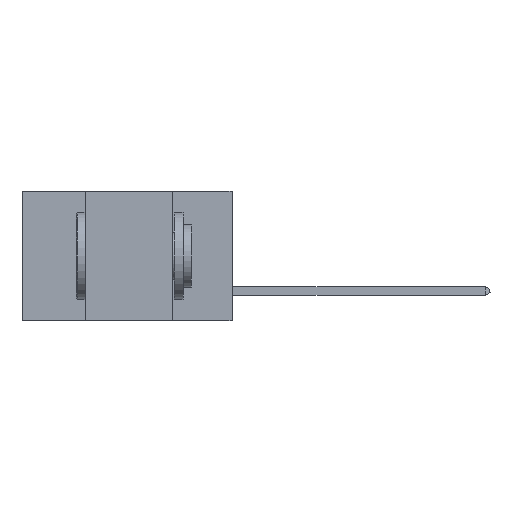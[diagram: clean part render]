
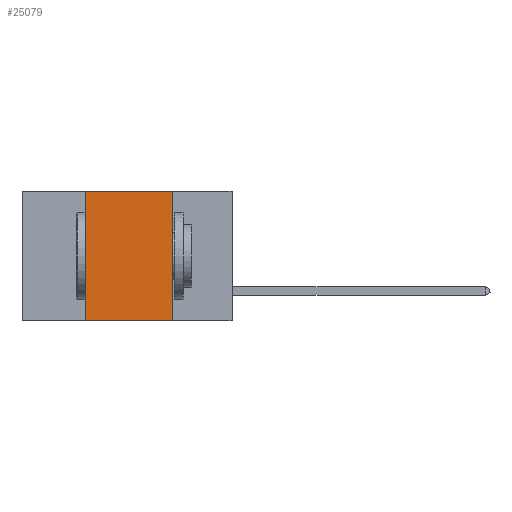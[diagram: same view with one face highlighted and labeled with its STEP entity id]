
A CAD part, left-side view. The second image highlights one B-rep face of the part: STEP entity #25079.
In plain terms, the highlighted planar face has unit normal (-1, 0, 0).
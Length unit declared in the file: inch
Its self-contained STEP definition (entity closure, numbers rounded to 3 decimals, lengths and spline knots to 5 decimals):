
#340 = CARTESIAN_POINT ( 'NONE',  ( 0., 0.6, -0.37 ) ) ;
#440 = LINE ( 'NONE', #6209, #5969 ) ;
#468 = CARTESIAN_POINT ( 'NONE',  ( 0., 0.17, 0. ) ) ;
#1213 = VERTEX_POINT ( 'NONE', #26043 ) ;
#1309 = LINE ( 'NONE', #468, #14433 ) ;
#3500 = VERTEX_POINT ( 'NONE', #23455 ) ;
#4245 = CARTESIAN_POINT ( 'NONE',  ( 0., 0.6, 0. ) ) ;
#5470 = CARTESIAN_POINT ( 'NONE',  ( 0., 0.17, -0.37 ) ) ;
#5969 = VECTOR ( 'NONE', #6392, 39.37008 ) ;
#6209 = CARTESIAN_POINT ( 'NONE',  ( 0., 0.42, 0. ) ) ;
#6392 = DIRECTION ( 'NONE',  ( 0., 0., 1. ) ) ;
#7601 = EDGE_CURVE ( 'NONE', #22792, #12223, #19669, .T. ) ;
#8671 = PLANE ( 'NONE',  #19554 ) ;
#9557 = EDGE_CURVE ( 'NONE', #22792, #3500, #440, .T. ) ;
#9713 = ORIENTED_EDGE ( 'NONE', *, *, #22068, .F. ) ;
#10502 = ORIENTED_EDGE ( 'NONE', *, *, #7601, .T. ) ;
#12223 = VERTEX_POINT ( 'NONE', #5470 ) ;
#13035 = VECTOR ( 'NONE', #13548, 39.37008 ) ;
#13548 = DIRECTION ( 'NONE',  ( 0., -1., 0. ) ) ;
#14433 = VECTOR ( 'NONE', #18175, 39.37008 ) ;
#17215 = ORIENTED_EDGE ( 'NONE', *, *, #21674, .F. ) ;
#18053 = ORIENTED_EDGE ( 'NONE', *, *, #9557, .F. ) ;
#18175 = DIRECTION ( 'NONE',  ( 0., 0., -1. ) ) ;
#19101 = VECTOR ( 'NONE', #26534, 39.37008 ) ;
#19554 = AXIS2_PLACEMENT_3D ( 'NONE', #4245, #21970, #19628 ) ;
#19628 = DIRECTION ( 'NONE',  ( 0., 0., -1. ) ) ;
#19669 = LINE ( 'NONE', #340, #13035 ) ;
#21271 = EDGE_LOOP ( 'NONE', ( #17215, #9713, #18053, #10502 ) ) ;
#21674 = EDGE_CURVE ( 'NONE', #1213, #12223, #1309, .T. ) ;
#21970 = DIRECTION ( 'NONE',  ( 1., 0., 0. ) ) ;
#22068 = EDGE_CURVE ( 'NONE', #3500, #1213, #25853, .T. ) ;
#22792 = VERTEX_POINT ( 'NONE', #24813 ) ;
#23455 = CARTESIAN_POINT ( 'NONE',  ( 0., 0.42, 0. ) ) ;
#24694 = CARTESIAN_POINT ( 'NONE',  ( 0., 0.6, 0. ) ) ;
#24813 = CARTESIAN_POINT ( 'NONE',  ( 0., 0.42, -0.37 ) ) ;
#25079 = ADVANCED_FACE ( 'NONE', ( #28265 ), #8671, .F. ) ;
#25853 = LINE ( 'NONE', #24694, #19101 ) ;
#26043 = CARTESIAN_POINT ( 'NONE',  ( 0., 0.17, 0. ) ) ;
#26534 = DIRECTION ( 'NONE',  ( 0., -1., 0. ) ) ;
#28265 = FACE_OUTER_BOUND ( 'NONE', #21271, .T. ) ;
